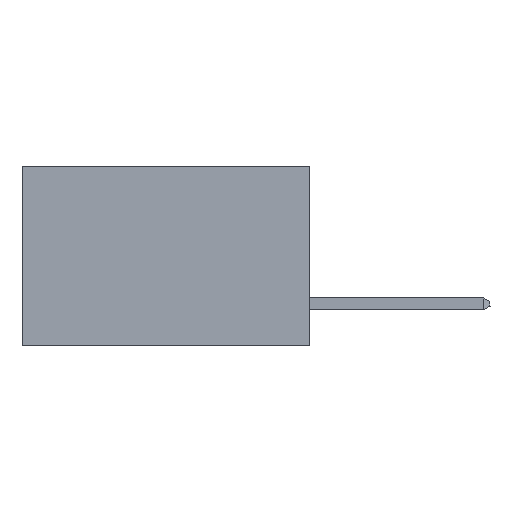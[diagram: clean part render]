
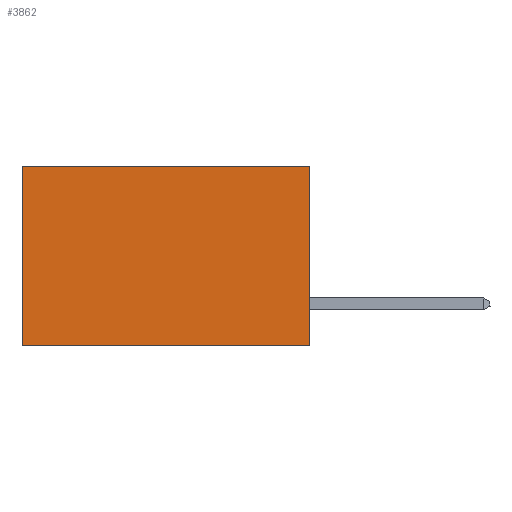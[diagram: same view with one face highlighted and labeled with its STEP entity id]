
A CAD part, left-side view. The second image highlights one B-rep face of the part: STEP entity #3862.
In plain terms, the highlighted planar face has unit normal (-1, 0, 0).
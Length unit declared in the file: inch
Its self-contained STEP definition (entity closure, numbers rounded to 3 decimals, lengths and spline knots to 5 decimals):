
#11 = CARTESIAN_POINT ( 'NONE',  ( 0.2875, 0., -0.375 ) ) ;
#1265 = CARTESIAN_POINT ( 'NONE',  ( 0.2875, 0.6, -0.375 ) ) ;
#1838 = EDGE_CURVE ( 'NONE', #2997, #5767, #8799, .T. ) ;
#2122 = CARTESIAN_POINT ( 'NONE',  ( 0.2875, 0., -0.375 ) ) ;
#2997 = VERTEX_POINT ( 'NONE', #20460 ) ;
#3236 = DIRECTION ( 'NONE',  ( 0., 1., 0. ) ) ;
#3665 = VERTEX_POINT ( 'NONE', #12056 ) ;
#3834 = PLANE ( 'NONE',  #5053 ) ;
#3862 = ADVANCED_FACE ( 'NONE', ( #10185 ), #3834, .F. ) ;
#4577 = VECTOR ( 'NONE', #16136, 39.37008 ) ;
#4704 = EDGE_CURVE ( 'NONE', #8790, #2997, #17577, .T. ) ;
#5053 = AXIS2_PLACEMENT_3D ( 'NONE', #13090, #8475, #19587 ) ;
#5767 = VERTEX_POINT ( 'NONE', #1265 ) ;
#6793 = EDGE_CURVE ( 'NONE', #8790, #3665, #14777, .T. ) ;
#6907 = CARTESIAN_POINT ( 'NONE',  ( 0.2875, 0.6, -0.375 ) ) ;
#7400 = ORIENTED_EDGE ( 'NONE', *, *, #1838, .F. ) ;
#7953 = CARTESIAN_POINT ( 'NONE',  ( 0.2875, 0., 0. ) ) ;
#8475 = DIRECTION ( 'NONE',  ( 1., 0., 0. ) ) ;
#8790 = VERTEX_POINT ( 'NONE', #14597 ) ;
#8799 = LINE ( 'NONE', #11, #19721 ) ;
#10185 = FACE_OUTER_BOUND ( 'NONE', #12516, .T. ) ;
#12056 = CARTESIAN_POINT ( 'NONE',  ( 0.2875, 0.6, 0. ) ) ;
#12516 = EDGE_LOOP ( 'NONE', ( #18977, #7400, #19821, #17661 ) ) ;
#13090 = CARTESIAN_POINT ( 'NONE',  ( 0.2875, 0., -0.375 ) ) ;
#14482 = EDGE_CURVE ( 'NONE', #3665, #5767, #16273, .T. ) ;
#14597 = CARTESIAN_POINT ( 'NONE',  ( 0.2875, 0., 0. ) ) ;
#14777 = LINE ( 'NONE', #7953, #4577 ) ;
#14887 = VECTOR ( 'NONE', #18083, 39.37008 ) ;
#14919 = DIRECTION ( 'NONE',  ( 0., 0., -1. ) ) ;
#16136 = DIRECTION ( 'NONE',  ( 0., 1., 0. ) ) ;
#16273 = LINE ( 'NONE', #6907, #20262 ) ;
#17577 = LINE ( 'NONE', #2122, #14887 ) ;
#17661 = ORIENTED_EDGE ( 'NONE', *, *, #6793, .T. ) ;
#18083 = DIRECTION ( 'NONE',  ( 0., 0., -1. ) ) ;
#18977 = ORIENTED_EDGE ( 'NONE', *, *, #14482, .T. ) ;
#19587 = DIRECTION ( 'NONE',  ( 0., 0., -1. ) ) ;
#19721 = VECTOR ( 'NONE', #3236, 39.37008 ) ;
#19821 = ORIENTED_EDGE ( 'NONE', *, *, #4704, .F. ) ;
#20262 = VECTOR ( 'NONE', #14919, 39.37008 ) ;
#20460 = CARTESIAN_POINT ( 'NONE',  ( 0.2875, 0., -0.375 ) ) ;
